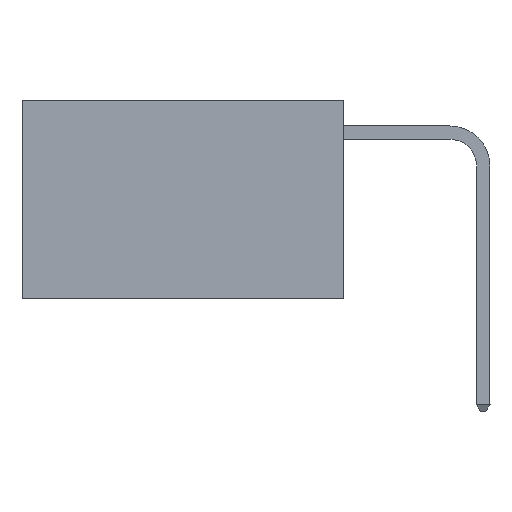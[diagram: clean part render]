
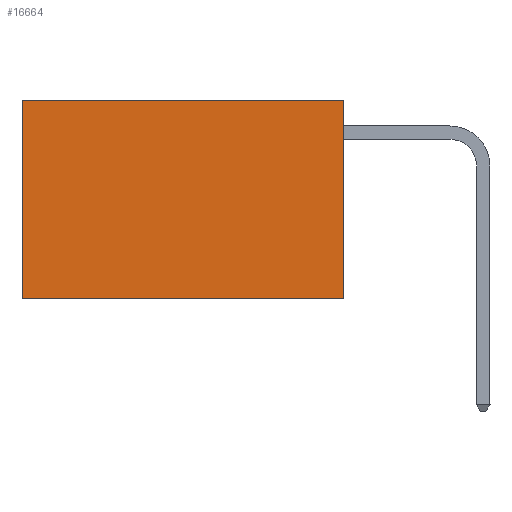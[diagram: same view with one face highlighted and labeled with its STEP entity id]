
A CAD part, left-side view. The second image highlights one B-rep face of the part: STEP entity #16664.
In plain terms, the highlighted planar face has unit normal (-1, 0, 0).
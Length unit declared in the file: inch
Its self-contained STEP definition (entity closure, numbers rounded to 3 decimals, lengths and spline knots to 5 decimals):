
#503 = CARTESIAN_POINT ( 'NONE',  ( 0.2625, 0., 0. ) ) ;
#1024 = ORIENTED_EDGE ( 'NONE', *, *, #7033, .F. ) ;
#1628 = DIRECTION ( 'NONE',  ( 0., 1., 0. ) ) ;
#1898 = VERTEX_POINT ( 'NONE', #12774 ) ;
#2292 = CARTESIAN_POINT ( 'NONE',  ( 0.2625, 0., -0.37 ) ) ;
#2461 = DIRECTION ( 'NONE',  ( 0., 0., -1. ) ) ;
#3136 = LINE ( 'NONE', #10205, #3588 ) ;
#3588 = VECTOR ( 'NONE', #1628, 39.37008 ) ;
#3608 = CARTESIAN_POINT ( 'NONE',  ( 0.2625, 0., 0. ) ) ;
#4240 = EDGE_CURVE ( 'NONE', #11247, #1898, #11296, .T. ) ;
#4854 = VERTEX_POINT ( 'NONE', #2292 ) ;
#4953 = DIRECTION ( 'NONE',  ( 0., 1., 0. ) ) ;
#5158 = VECTOR ( 'NONE', #2461, 39.37008 ) ;
#5223 = ORIENTED_EDGE ( 'NONE', *, *, #13574, .T. ) ;
#5426 = VECTOR ( 'NONE', #9878, 39.37008 ) ;
#7033 = EDGE_CURVE ( 'NONE', #4854, #1898, #3136, .T. ) ;
#7926 = CARTESIAN_POINT ( 'NONE',  ( 0.2625, 0.6, 0. ) ) ;
#8060 = LINE ( 'NONE', #503, #13572 ) ;
#8527 = VERTEX_POINT ( 'NONE', #3608 ) ;
#8704 = EDGE_CURVE ( 'NONE', #8527, #4854, #11056, .T. ) ;
#9548 = AXIS2_PLACEMENT_3D ( 'NONE', #14164, #12570, #9664 ) ;
#9664 = DIRECTION ( 'NONE',  ( 0., 0., -1. ) ) ;
#9750 = PLANE ( 'NONE',  #9548 ) ;
#9878 = DIRECTION ( 'NONE',  ( 0., 0., -1. ) ) ;
#10205 = CARTESIAN_POINT ( 'NONE',  ( 0.2625, 0., -0.37 ) ) ;
#11056 = LINE ( 'NONE', #15381, #5158 ) ;
#11247 = VERTEX_POINT ( 'NONE', #7926 ) ;
#11296 = LINE ( 'NONE', #17040, #5426 ) ;
#12570 = DIRECTION ( 'NONE',  ( 1., 0., 0. ) ) ;
#12774 = CARTESIAN_POINT ( 'NONE',  ( 0.2625, 0.6, -0.37 ) ) ;
#13008 = EDGE_LOOP ( 'NONE', ( #14022, #1024, #14497, #5223 ) ) ;
#13572 = VECTOR ( 'NONE', #4953, 39.37008 ) ;
#13574 = EDGE_CURVE ( 'NONE', #8527, #11247, #8060, .T. ) ;
#14022 = ORIENTED_EDGE ( 'NONE', *, *, #4240, .T. ) ;
#14164 = CARTESIAN_POINT ( 'NONE',  ( 0.2625, 0., 0. ) ) ;
#14497 = ORIENTED_EDGE ( 'NONE', *, *, #8704, .F. ) ;
#15381 = CARTESIAN_POINT ( 'NONE',  ( 0.2625, 0., 0. ) ) ;
#16664 = ADVANCED_FACE ( 'NONE', ( #17008 ), #9750, .F. ) ;
#17008 = FACE_OUTER_BOUND ( 'NONE', #13008, .T. ) ;
#17040 = CARTESIAN_POINT ( 'NONE',  ( 0.2625, 0.6, 0. ) ) ;
